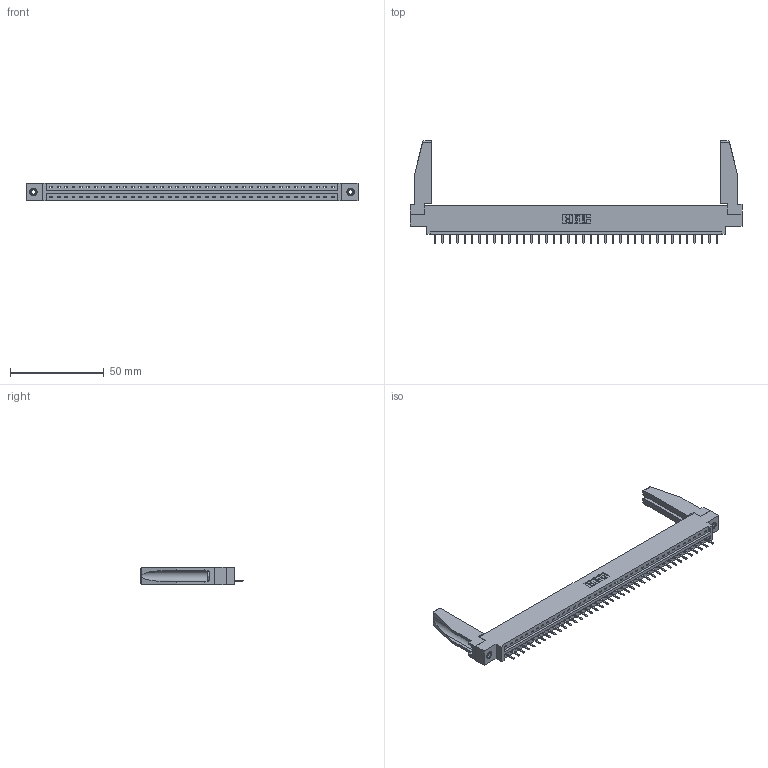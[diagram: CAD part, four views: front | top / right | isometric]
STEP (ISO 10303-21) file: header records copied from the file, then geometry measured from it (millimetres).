
FILE_DESCRIPTION (( 'STEP AP203' ), '1' );
FILE_NAME ('387-039-520-678.STEP', '2019-10-04T16:53:57', ( '' ), ( '' ), 'SwSTEP 2.0', 'SolidWorks 2016', '' );
FILE_SCHEMA (( 'CONFIG_CONTROL_DESIGN' ));
Length unit declared in the file: inch
Products named in the file (5): 337 Part_0.170 Offset - 0.156 Dia-TI; 307-220-078; 345-292-001_345-293-120; 387-039-520-678; 345-250-001_345-250-001-102
Assembly tree (44 placements, depth 2):
  387-039-520-678
    337 Part_0.170 Offset - 0.156 Dia-TI
    345-292-001_345-293-120  x39
    345-250-001_345-250-001-102  x2
    307-220-078  x2
Bounding box: 177.55 x 54.82 x 9.4 mm (x, y, z)
Volume: 22179 mm3; surface area: 22305.1 mm2
Topology: 44 solids, 44 shells, 2822 faces, 8297 edges, 5418 vertices
Faces by surface type: plane 2030, cylinder 776, cone 12, torus 4
Entity records: 32064 total; most frequent: CARTESIAN_POINT 5589, ORIENTED_EDGE 5508, DIRECTION 4708, EDGE_CURVE 2754, LINE 2584, VECTOR 2584, VERTEX_POINT 1828, AXIS2_PLACEMENT_3D 1062
